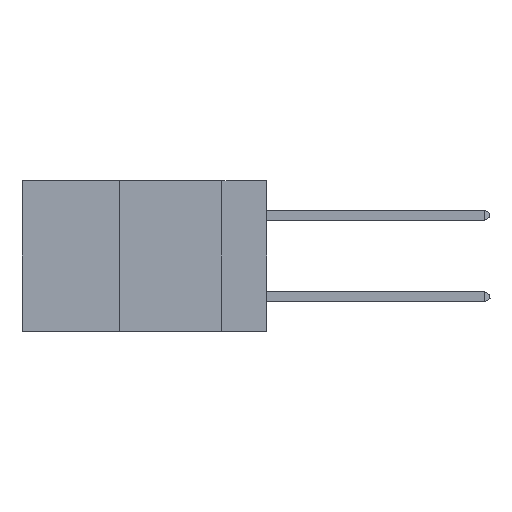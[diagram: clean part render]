
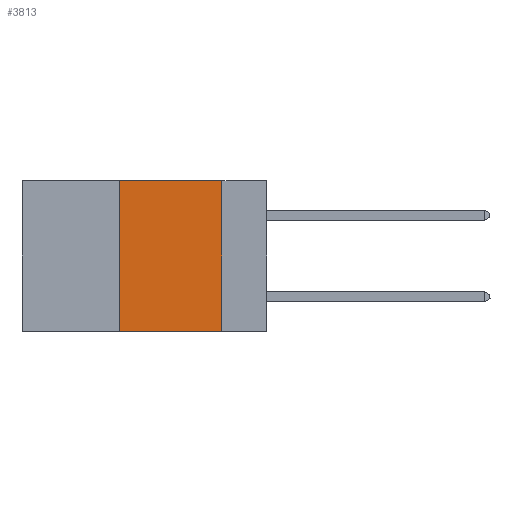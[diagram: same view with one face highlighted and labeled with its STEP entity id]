
A CAD part, left-side view. The second image highlights one B-rep face of the part: STEP entity #3813.
In plain terms, the highlighted planar face has unit normal (-1, 0, 0).
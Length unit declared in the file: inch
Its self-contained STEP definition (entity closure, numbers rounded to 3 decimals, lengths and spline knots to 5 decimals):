
#58 = CARTESIAN_POINT ( 'NONE',  ( 0., 0.6, 0. ) ) ;
#421 = EDGE_LOOP ( 'NONE', ( #15038, #3208, #7046, #2066 ) ) ;
#697 = EDGE_CURVE ( 'NONE', #2148, #3432, #5992, .T. ) ;
#1185 = DIRECTION ( 'NONE',  ( 1., 0., 0. ) ) ;
#1344 = VECTOR ( 'NONE', #15016, 39.37008 ) ;
#1506 = VERTEX_POINT ( 'NONE', #7339 ) ;
#2066 = ORIENTED_EDGE ( 'NONE', *, *, #6822, .T. ) ;
#2148 = VERTEX_POINT ( 'NONE', #11447 ) ;
#2295 = EDGE_CURVE ( 'NONE', #1506, #2148, #13438, .T. ) ;
#3208 = ORIENTED_EDGE ( 'NONE', *, *, #2295, .F. ) ;
#3432 = VERTEX_POINT ( 'NONE', #12868 ) ;
#3601 = LINE ( 'NONE', #7921, #5417 ) ;
#3813 = ADVANCED_FACE ( 'NONE', ( #13581 ), #5866, .F. ) ;
#3880 = CARTESIAN_POINT ( 'NONE',  ( 0., 0.36, 0. ) ) ;
#5417 = VECTOR ( 'NONE', #9174, 39.37008 ) ;
#5866 = PLANE ( 'NONE',  #7222 ) ;
#5972 = CARTESIAN_POINT ( 'NONE',  ( 0., 0.6, 0. ) ) ;
#5992 = LINE ( 'NONE', #8002, #1344 ) ;
#6822 = EDGE_CURVE ( 'NONE', #9905, #3432, #3601, .T. ) ;
#7000 = DIRECTION ( 'NONE',  ( 0., -1., 0. ) ) ;
#7046 = ORIENTED_EDGE ( 'NONE', *, *, #8089, .F. ) ;
#7222 = AXIS2_PLACEMENT_3D ( 'NONE', #5972, #1185, #8161 ) ;
#7339 = CARTESIAN_POINT ( 'NONE',  ( 0., 0.36, 0. ) ) ;
#7666 = CARTESIAN_POINT ( 'NONE',  ( 0., 0.36, -0.37 ) ) ;
#7921 = CARTESIAN_POINT ( 'NONE',  ( 0., 0.6, -0.37 ) ) ;
#8002 = CARTESIAN_POINT ( 'NONE',  ( 0., 0.11, 0. ) ) ;
#8089 = EDGE_CURVE ( 'NONE', #9905, #1506, #12672, .T. ) ;
#8161 = DIRECTION ( 'NONE',  ( 0., 0., -1. ) ) ;
#9174 = DIRECTION ( 'NONE',  ( 0., -1., 0. ) ) ;
#9773 = DIRECTION ( 'NONE',  ( 0., 0., 1. ) ) ;
#9905 = VERTEX_POINT ( 'NONE', #7666 ) ;
#11447 = CARTESIAN_POINT ( 'NONE',  ( 0., 0.11, 0. ) ) ;
#12497 = VECTOR ( 'NONE', #7000, 39.37008 ) ;
#12672 = LINE ( 'NONE', #3880, #13810 ) ;
#12868 = CARTESIAN_POINT ( 'NONE',  ( 0., 0.11, -0.37 ) ) ;
#13438 = LINE ( 'NONE', #58, #12497 ) ;
#13581 = FACE_OUTER_BOUND ( 'NONE', #421, .T. ) ;
#13810 = VECTOR ( 'NONE', #9773, 39.37008 ) ;
#15016 = DIRECTION ( 'NONE',  ( 0., 0., -1. ) ) ;
#15038 = ORIENTED_EDGE ( 'NONE', *, *, #697, .F. ) ;
